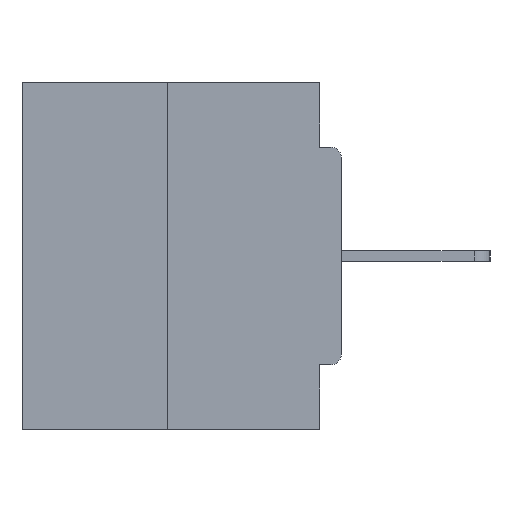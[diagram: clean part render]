
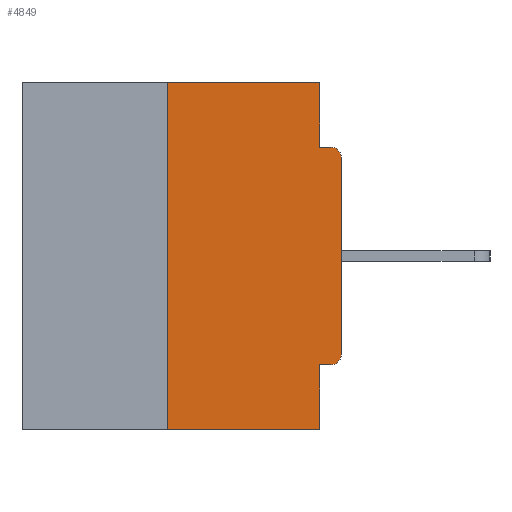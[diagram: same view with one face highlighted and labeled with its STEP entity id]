
A CAD part, left-side view. The second image highlights one B-rep face of the part: STEP entity #4849.
In plain terms, the highlighted planar face has unit normal (-1, 0, 0).
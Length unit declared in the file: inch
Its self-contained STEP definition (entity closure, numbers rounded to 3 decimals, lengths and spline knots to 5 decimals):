
#190 = EDGE_LOOP ( 'NONE', ( #16285, #4071, #27581, #21610, #8393, #2159, #20759, #3061, #20795, #17723 ) ) ;
#874 = VECTOR ( 'NONE', #4548, 39.37008 ) ;
#1041 = VERTEX_POINT ( 'NONE', #26425 ) ;
#1498 = LINE ( 'NONE', #13735, #874 ) ;
#1515 = DIRECTION ( 'NONE',  ( 0., 1., 0. ) ) ;
#1624 = EDGE_CURVE ( 'NONE', #9725, #7041, #17515, .T. ) ;
#2108 = CARTESIAN_POINT ( 'NONE',  ( 0., 0.015, -0.1085 ) ) ;
#2159 = ORIENTED_EDGE ( 'NONE', *, *, #4490, .T. ) ;
#2183 = EDGE_CURVE ( 'NONE', #23492, #3960, #29703, .T. ) ;
#2399 = DIRECTION ( 'NONE',  ( 0., 0., -1. ) ) ;
#3061 = ORIENTED_EDGE ( 'NONE', *, *, #24273, .T. ) ;
#3909 = CARTESIAN_POINT ( 'NONE',  ( 0., 0.015, -0.0935 ) ) ;
#3960 = VERTEX_POINT ( 'NONE', #11574 ) ;
#3976 = VERTEX_POINT ( 'NONE', #12485 ) ;
#4071 = ORIENTED_EDGE ( 'NONE', *, *, #5789, .F. ) ;
#4341 = LINE ( 'NONE', #9097, #20428 ) ;
#4490 = EDGE_CURVE ( 'NONE', #23492, #27524, #27508, .T. ) ;
#4548 = DIRECTION ( 'NONE',  ( 0., 0., -1. ) ) ;
#4849 = ADVANCED_FACE ( 'NONE', ( #14854 ), #5197, .F. ) ;
#5197 = PLANE ( 'NONE',  #23389 ) ;
#5723 = LINE ( 'NONE', #10477, #17561 ) ;
#5789 = EDGE_CURVE ( 'NONE', #21716, #10060, #20560, .T. ) ;
#6034 = CARTESIAN_POINT ( 'NONE',  ( 0., 0., -0.3915 ) ) ;
#7041 = VERTEX_POINT ( 'NONE', #3909 ) ;
#7651 = DIRECTION ( 'NONE',  ( 1., 0., 0. ) ) ;
#7700 = VECTOR ( 'NONE', #17301, 39.37008 ) ;
#8393 = ORIENTED_EDGE ( 'NONE', *, *, #2183, .F. ) ;
#8727 = EDGE_CURVE ( 'NONE', #27524, #1041, #26955, .T. ) ;
#8848 = EDGE_CURVE ( 'NONE', #3960, #3976, #1498, .T. ) ;
#9097 = CARTESIAN_POINT ( 'NONE',  ( 0., 0.46, 0. ) ) ;
#9725 = VERTEX_POINT ( 'NONE', #14698 ) ;
#9918 = CARTESIAN_POINT ( 'NONE',  ( 0., 0.031, 0. ) ) ;
#10060 = VERTEX_POINT ( 'NONE', #18355 ) ;
#10453 = DIRECTION ( 'NONE',  ( 0., -1., 0. ) ) ;
#10477 = CARTESIAN_POINT ( 'NONE',  ( 0., 0.46, -0.5 ) ) ;
#10890 = CARTESIAN_POINT ( 'NONE',  ( 0., 0.015, -0.4065 ) ) ;
#11525 = DIRECTION ( 'NONE',  ( 0., -1., 0. ) ) ;
#11574 = CARTESIAN_POINT ( 'NONE',  ( 0., 0.031, -0.4065 ) ) ;
#12047 = LINE ( 'NONE', #9918, #13657 ) ;
#12485 = CARTESIAN_POINT ( 'NONE',  ( 0., 0.031, -0.5 ) ) ;
#13186 = CARTESIAN_POINT ( 'NONE',  ( 0., 0.25, 0. ) ) ;
#13197 = DIRECTION ( 'NONE',  ( 0., 0., -1. ) ) ;
#13657 = VECTOR ( 'NONE', #2399, 39.37008 ) ;
#13735 = CARTESIAN_POINT ( 'NONE',  ( 0., 0.031, -0.5 ) ) ;
#14698 = CARTESIAN_POINT ( 'NONE',  ( 0., 0.031, -0.0935 ) ) ;
#14854 = FACE_OUTER_BOUND ( 'NONE', #190, .T. ) ;
#16239 = AXIS2_PLACEMENT_3D ( 'NONE', #21959, #24850, #13197 ) ;
#16285 = ORIENTED_EDGE ( 'NONE', *, *, #16687, .F. ) ;
#16687 = EDGE_CURVE ( 'NONE', #10060, #27516, #4341, .T. ) ;
#17231 = CARTESIAN_POINT ( 'NONE',  ( 0., 0.25, -0.5 ) ) ;
#17301 = DIRECTION ( 'NONE',  ( 0., 0., 1. ) ) ;
#17376 = VECTOR ( 'NONE', #1515, 39.37008 ) ;
#17515 = LINE ( 'NONE', #27015, #24016 ) ;
#17561 = VECTOR ( 'NONE', #19829, 39.37008 ) ;
#17723 = ORIENTED_EDGE ( 'NONE', *, *, #27989, .F. ) ;
#18355 = CARTESIAN_POINT ( 'NONE',  ( 0., 0.25, 0. ) ) ;
#19829 = DIRECTION ( 'NONE',  ( 0., -1., 0. ) ) ;
#20428 = VECTOR ( 'NONE', #11525, 39.37008 ) ;
#20560 = LINE ( 'NONE', #13186, #24624 ) ;
#20759 = ORIENTED_EDGE ( 'NONE', *, *, #8727, .T. ) ;
#20795 = ORIENTED_EDGE ( 'NONE', *, *, #1624, .F. ) ;
#20802 = DIRECTION ( 'NONE',  ( -1., 0., 0. ) ) ;
#21610 = ORIENTED_EDGE ( 'NONE', *, *, #8848, .F. ) ;
#21716 = VERTEX_POINT ( 'NONE', #17231 ) ;
#21801 = AXIS2_PLACEMENT_3D ( 'NONE', #2108, #20802, #23545 ) ;
#21959 = CARTESIAN_POINT ( 'NONE',  ( 0., 0.015, -0.3915 ) ) ;
#22550 = DIRECTION ( 'NONE',  ( 0., 0., 1. ) ) ;
#23389 = AXIS2_PLACEMENT_3D ( 'NONE', #24188, #7651, #28637 ) ;
#23492 = VERTEX_POINT ( 'NONE', #10890 ) ;
#23545 = DIRECTION ( 'NONE',  ( 0., 0., -1. ) ) ;
#24016 = VECTOR ( 'NONE', #10453, 39.37008 ) ;
#24188 = CARTESIAN_POINT ( 'NONE',  ( 0., 0.46, 0. ) ) ;
#24273 = EDGE_CURVE ( 'NONE', #1041, #7041, #30110, .T. ) ;
#24624 = VECTOR ( 'NONE', #22550, 39.37008 ) ;
#24778 = CARTESIAN_POINT ( 'NONE',  ( 0., 0., 0. ) ) ;
#24797 = CARTESIAN_POINT ( 'NONE',  ( 0., 0., -0.4065 ) ) ;
#24850 = DIRECTION ( 'NONE',  ( -1., 0., 0. ) ) ;
#26425 = CARTESIAN_POINT ( 'NONE',  ( 0., 0., -0.1085 ) ) ;
#26955 = LINE ( 'NONE', #24778, #7700 ) ;
#27015 = CARTESIAN_POINT ( 'NONE',  ( 0., 0., -0.0935 ) ) ;
#27391 = EDGE_CURVE ( 'NONE', #21716, #3976, #5723, .T. ) ;
#27508 = CIRCLE ( 'NONE', #16239, 0.015 ) ;
#27516 = VERTEX_POINT ( 'NONE', #27632 ) ;
#27524 = VERTEX_POINT ( 'NONE', #6034 ) ;
#27581 = ORIENTED_EDGE ( 'NONE', *, *, #27391, .T. ) ;
#27632 = CARTESIAN_POINT ( 'NONE',  ( 0., 0.031, 0. ) ) ;
#27989 = EDGE_CURVE ( 'NONE', #27516, #9725, #12047, .T. ) ;
#28637 = DIRECTION ( 'NONE',  ( 0., 0., -1. ) ) ;
#29703 = LINE ( 'NONE', #24797, #17376 ) ;
#30110 = CIRCLE ( 'NONE', #21801, 0.015 ) ;
